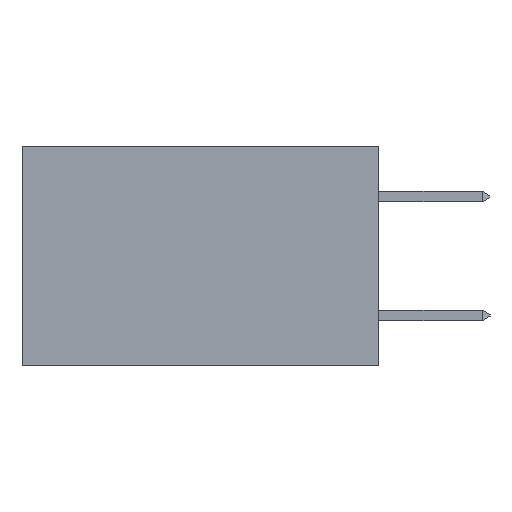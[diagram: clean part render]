
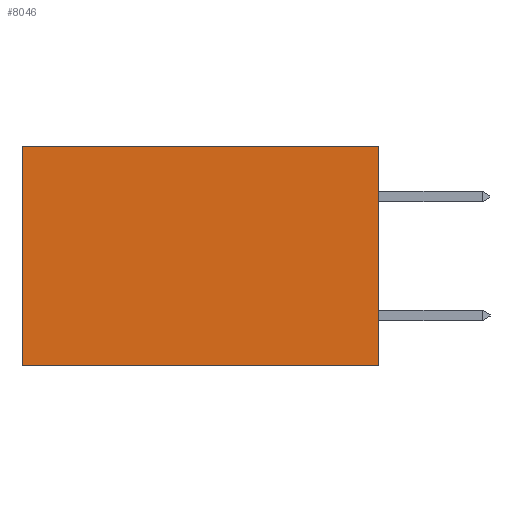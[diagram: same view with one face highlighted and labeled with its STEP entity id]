
A CAD part, left-side view. The second image highlights one B-rep face of the part: STEP entity #8046.
In plain terms, the highlighted planar face has unit normal (-1, 0, 0).
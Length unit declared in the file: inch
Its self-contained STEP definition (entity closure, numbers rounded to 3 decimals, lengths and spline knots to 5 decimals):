
#107 = EDGE_CURVE ( 'NONE', #7070, #3782, #2533, .T. ) ;
#202 = EDGE_CURVE ( 'NONE', #9933, #3782, #5442, .T. ) ;
#224 = EDGE_LOOP ( 'NONE', ( #7337, #8734, #4817, #4756 ) ) ;
#258 = DIRECTION ( 'NONE',  ( 0., 1., 0. ) ) ;
#610 = CARTESIAN_POINT ( 'NONE',  ( 0.2615, 0., -0.37 ) ) ;
#1191 = CARTESIAN_POINT ( 'NONE',  ( 0.2615, 0., -0.37 ) ) ;
#1515 = CARTESIAN_POINT ( 'NONE',  ( 0.2615, 0.6, 0. ) ) ;
#2429 = FACE_OUTER_BOUND ( 'NONE', #224, .T. ) ;
#2533 = LINE ( 'NONE', #6330, #8924 ) ;
#3016 = DIRECTION ( 'NONE',  ( 0., 0., -1. ) ) ;
#3220 = DIRECTION ( 'NONE',  ( 0., 0., -1. ) ) ;
#3489 = EDGE_CURVE ( 'NONE', #10612, #9933, #9419, .T. ) ;
#3732 = VECTOR ( 'NONE', #5416, 39.37008 ) ;
#3748 = CARTESIAN_POINT ( 'NONE',  ( 0.2615, 0.6, -0.37 ) ) ;
#3782 = VERTEX_POINT ( 'NONE', #3748 ) ;
#3964 = CARTESIAN_POINT ( 'NONE',  ( 0.2615, 0., 0. ) ) ;
#4756 = ORIENTED_EDGE ( 'NONE', *, *, #10316, .T. ) ;
#4804 = AXIS2_PLACEMENT_3D ( 'NONE', #1191, #8052, #3016 ) ;
#4817 = ORIENTED_EDGE ( 'NONE', *, *, #3489, .F. ) ;
#5023 = VECTOR ( 'NONE', #8610, 39.37008 ) ;
#5416 = DIRECTION ( 'NONE',  ( 0., 1., 0. ) ) ;
#5442 = LINE ( 'NONE', #7540, #7407 ) ;
#6006 = LINE ( 'NONE', #8706, #3732 ) ;
#6330 = CARTESIAN_POINT ( 'NONE',  ( 0.2615, 0.6, -0.37 ) ) ;
#7070 = VERTEX_POINT ( 'NONE', #1515 ) ;
#7207 = PLANE ( 'NONE',  #4804 ) ;
#7337 = ORIENTED_EDGE ( 'NONE', *, *, #107, .T. ) ;
#7407 = VECTOR ( 'NONE', #258, 39.37008 ) ;
#7540 = CARTESIAN_POINT ( 'NONE',  ( 0.2615, 0., -0.37 ) ) ;
#8046 = ADVANCED_FACE ( 'NONE', ( #2429 ), #7207, .F. ) ;
#8052 = DIRECTION ( 'NONE',  ( 1., 0., 0. ) ) ;
#8575 = CARTESIAN_POINT ( 'NONE',  ( 0.2615, 0., -0.37 ) ) ;
#8610 = DIRECTION ( 'NONE',  ( 0., 0., -1. ) ) ;
#8706 = CARTESIAN_POINT ( 'NONE',  ( 0.2615, 0., 0. ) ) ;
#8734 = ORIENTED_EDGE ( 'NONE', *, *, #202, .F. ) ;
#8924 = VECTOR ( 'NONE', #3220, 39.37008 ) ;
#9419 = LINE ( 'NONE', #8575, #5023 ) ;
#9933 = VERTEX_POINT ( 'NONE', #610 ) ;
#10316 = EDGE_CURVE ( 'NONE', #10612, #7070, #6006, .T. ) ;
#10612 = VERTEX_POINT ( 'NONE', #3964 ) ;
